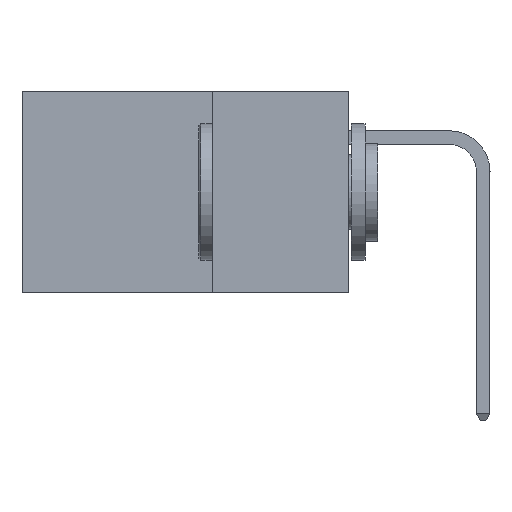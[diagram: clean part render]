
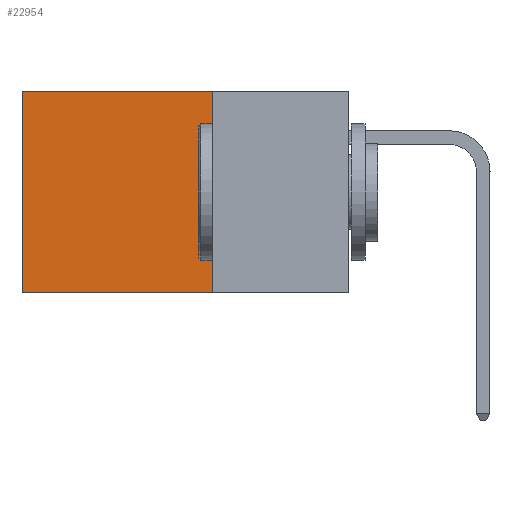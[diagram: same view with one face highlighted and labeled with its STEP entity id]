
A CAD part, left-side view. The second image highlights one B-rep face of the part: STEP entity #22954.
In plain terms, the highlighted planar face has unit normal (-1, 0, 0).
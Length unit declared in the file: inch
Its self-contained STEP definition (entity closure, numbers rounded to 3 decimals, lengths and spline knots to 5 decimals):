
#715 = CARTESIAN_POINT ( 'NONE',  ( 0.2875, 0.25, 0. ) ) ;
#1928 = EDGE_LOOP ( 'NONE', ( #43157, #5602, #6557, #9190 ) ) ;
#2350 = LINE ( 'NONE', #25588, #22754 ) ;
#5602 = ORIENTED_EDGE ( 'NONE', *, *, #35411, .F. ) ;
#6316 = EDGE_CURVE ( 'NONE', #8362, #21087, #39471, .T. ) ;
#6557 = ORIENTED_EDGE ( 'NONE', *, *, #9767, .F. ) ;
#6768 = DIRECTION ( 'NONE',  ( 0., 1., 0. ) ) ;
#7897 = CARTESIAN_POINT ( 'NONE',  ( 0.2875, 0.6, -0.37 ) ) ;
#8176 = DIRECTION ( 'NONE',  ( 0., 1., 0. ) ) ;
#8362 = VERTEX_POINT ( 'NONE', #42042 ) ;
#8924 = CARTESIAN_POINT ( 'NONE',  ( 0.2875, 0.25, -0.37 ) ) ;
#9190 = ORIENTED_EDGE ( 'NONE', *, *, #42951, .T. ) ;
#9644 = DIRECTION ( 'NONE',  ( 1., 0., 0. ) ) ;
#9767 = EDGE_CURVE ( 'NONE', #17601, #19729, #22718, .T. ) ;
#11139 = LINE ( 'NONE', #26893, #42448 ) ;
#11755 = CARTESIAN_POINT ( 'NONE',  ( 0.2875, 0.25, 0. ) ) ;
#14321 = AXIS2_PLACEMENT_3D ( 'NONE', #43301, #9644, #41625 ) ;
#17601 = VERTEX_POINT ( 'NONE', #11755 ) ;
#19729 = VERTEX_POINT ( 'NONE', #8924 ) ;
#19791 = CARTESIAN_POINT ( 'NONE',  ( 0.2875, 0.6, 0. ) ) ;
#21087 = VERTEX_POINT ( 'NONE', #7897 ) ;
#22153 = VECTOR ( 'NONE', #42172, 39.37008 ) ;
#22718 = LINE ( 'NONE', #715, #22153 ) ;
#22754 = VECTOR ( 'NONE', #8176, 39.37008 ) ;
#22954 = ADVANCED_FACE ( 'NONE', ( #30180 ), #25446, .F. ) ;
#25446 = PLANE ( 'NONE',  #14321 ) ;
#25588 = CARTESIAN_POINT ( 'NONE',  ( 0.2875, 0.25, -0.37 ) ) ;
#26893 = CARTESIAN_POINT ( 'NONE',  ( 0.2875, 0.25, 0. ) ) ;
#30180 = FACE_OUTER_BOUND ( 'NONE', #1928, .T. ) ;
#31354 = VECTOR ( 'NONE', #40651, 39.37008 ) ;
#35411 = EDGE_CURVE ( 'NONE', #19729, #21087, #2350, .T. ) ;
#39471 = LINE ( 'NONE', #19791, #31354 ) ;
#40651 = DIRECTION ( 'NONE',  ( 0., 0., -1. ) ) ;
#41625 = DIRECTION ( 'NONE',  ( 0., 0., -1. ) ) ;
#42042 = CARTESIAN_POINT ( 'NONE',  ( 0.2875, 0.6, 0. ) ) ;
#42172 = DIRECTION ( 'NONE',  ( 0., 0., -1. ) ) ;
#42448 = VECTOR ( 'NONE', #6768, 39.37008 ) ;
#42951 = EDGE_CURVE ( 'NONE', #17601, #8362, #11139, .T. ) ;
#43157 = ORIENTED_EDGE ( 'NONE', *, *, #6316, .T. ) ;
#43301 = CARTESIAN_POINT ( 'NONE',  ( 0.2875, 0.25, 0. ) ) ;
